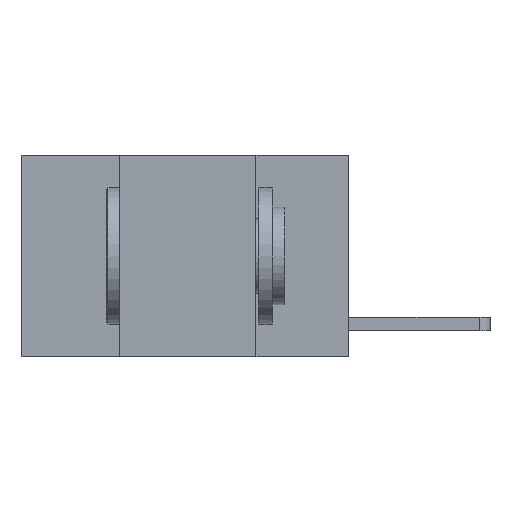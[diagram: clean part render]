
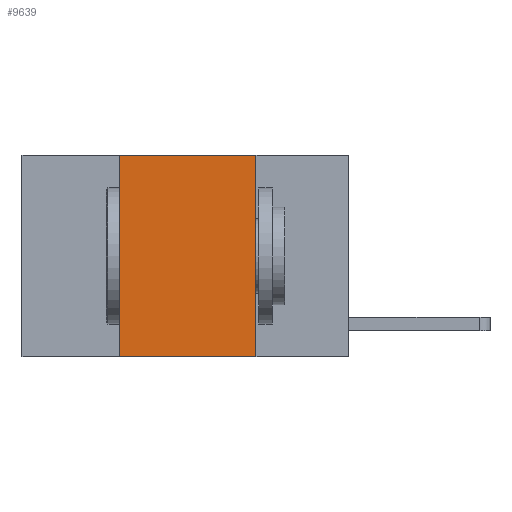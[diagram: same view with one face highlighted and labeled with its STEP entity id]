
A CAD part, left-side view. The second image highlights one B-rep face of the part: STEP entity #9639.
In plain terms, the highlighted planar face has unit normal (-1, 0, 0).
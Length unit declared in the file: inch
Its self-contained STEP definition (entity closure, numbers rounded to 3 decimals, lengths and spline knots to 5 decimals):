
#327 = CARTESIAN_POINT ( 'NONE',  ( 0., 0.6, -0.37 ) ) ;
#406 = DIRECTION ( 'NONE',  ( 0., -1., 0. ) ) ;
#598 = VECTOR ( 'NONE', #6170, 39.37008 ) ;
#740 = CARTESIAN_POINT ( 'NONE',  ( 0., 0.6, 0. ) ) ;
#1158 = DIRECTION ( 'NONE',  ( 0., 0., 1. ) ) ;
#1188 = CARTESIAN_POINT ( 'NONE',  ( 0., 0.42, 0. ) ) ;
#1560 = VECTOR ( 'NONE', #9443, 39.37008 ) ;
#1655 = DIRECTION ( 'NONE',  ( 1., 0., 0. ) ) ;
#2060 = AXIS2_PLACEMENT_3D ( 'NONE', #740, #1655, #7501 ) ;
#2121 = LINE ( 'NONE', #1188, #10542 ) ;
#3105 = VERTEX_POINT ( 'NONE', #8478 ) ;
#3613 = ORIENTED_EDGE ( 'NONE', *, *, #6089, .F. ) ;
#4196 = EDGE_CURVE ( 'NONE', #5073, #3105, #7365, .T. ) ;
#4488 = EDGE_CURVE ( 'NONE', #4516, #7209, #4833, .T. ) ;
#4512 = ORIENTED_EDGE ( 'NONE', *, *, #4196, .F. ) ;
#4516 = VERTEX_POINT ( 'NONE', #10658 ) ;
#4783 = ORIENTED_EDGE ( 'NONE', *, *, #5565, .F. ) ;
#4833 = LINE ( 'NONE', #327, #9099 ) ;
#5073 = VERTEX_POINT ( 'NONE', #5809 ) ;
#5136 = ORIENTED_EDGE ( 'NONE', *, *, #4488, .T. ) ;
#5565 = EDGE_CURVE ( 'NONE', #4516, #5073, #2121, .T. ) ;
#5809 = CARTESIAN_POINT ( 'NONE',  ( 0., 0.42, 0. ) ) ;
#6089 = EDGE_CURVE ( 'NONE', #3105, #7209, #8450, .T. ) ;
#6170 = DIRECTION ( 'NONE',  ( 0., -1., 0. ) ) ;
#6681 = PLANE ( 'NONE',  #2060 ) ;
#6859 = CARTESIAN_POINT ( 'NONE',  ( 0., 0.6, 0. ) ) ;
#7209 = VERTEX_POINT ( 'NONE', #7478 ) ;
#7365 = LINE ( 'NONE', #6859, #598 ) ;
#7373 = EDGE_LOOP ( 'NONE', ( #3613, #4512, #4783, #5136 ) ) ;
#7478 = CARTESIAN_POINT ( 'NONE',  ( 0., 0.17, -0.37 ) ) ;
#7501 = DIRECTION ( 'NONE',  ( 0., 0., -1. ) ) ;
#8450 = LINE ( 'NONE', #9705, #1560 ) ;
#8478 = CARTESIAN_POINT ( 'NONE',  ( 0., 0.17, 0. ) ) ;
#9099 = VECTOR ( 'NONE', #406, 39.37008 ) ;
#9443 = DIRECTION ( 'NONE',  ( 0., 0., -1. ) ) ;
#9639 = ADVANCED_FACE ( 'NONE', ( #9873 ), #6681, .F. ) ;
#9705 = CARTESIAN_POINT ( 'NONE',  ( 0., 0.17, 0. ) ) ;
#9873 = FACE_OUTER_BOUND ( 'NONE', #7373, .T. ) ;
#10542 = VECTOR ( 'NONE', #1158, 39.37008 ) ;
#10658 = CARTESIAN_POINT ( 'NONE',  ( 0., 0.42, -0.37 ) ) ;
